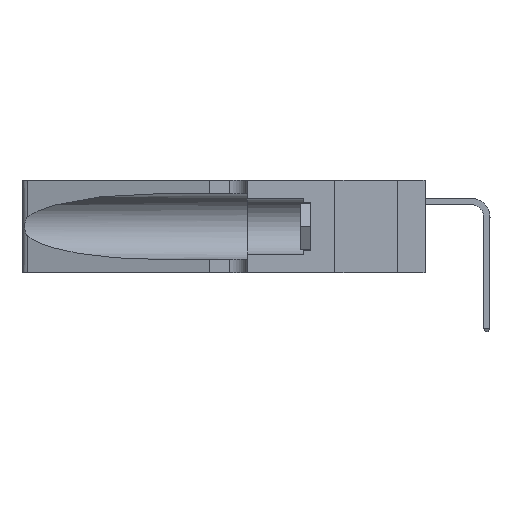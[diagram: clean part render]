
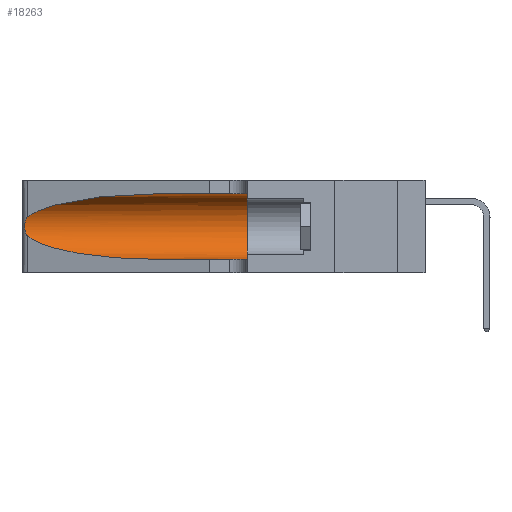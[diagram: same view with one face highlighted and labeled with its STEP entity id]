
A CAD part, left-side view. The second image highlights one B-rep face of the part: STEP entity #18263.
In plain terms, the highlighted cylindrical face has radius 3.308 mm (diameter 6.617 mm), a partial arc.
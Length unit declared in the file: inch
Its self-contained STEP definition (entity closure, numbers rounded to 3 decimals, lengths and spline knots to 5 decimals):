
#2516 = CARTESIAN_POINT ( 'NONE',  ( 0.26075, 1.23896, 0.19203 ) ) ;
#4364 = VERTEX_POINT ( 'NONE', #32372 ) ;
#5464 = CARTESIAN_POINT ( 'NONE',  ( 0.25487, 1.22718, 0.14631 ) ) ;
#6122 = CARTESIAN_POINT ( 'NONE',  ( 0.26017, 1.23833, 0.17102 ) ) ;
#6184 = VERTEX_POINT ( 'NONE', #35176 ) ;
#6889 = CARTESIAN_POINT ( 'NONE',  ( 0.25487, 1.22718, 0.22369 ) ) ;
#7585 = EDGE_CURVE ( 'NONE', #8695, #30227, #9266, .T. ) ;
#8695 = VERTEX_POINT ( 'NONE', #9347 ) ;
#8862 = CARTESIAN_POINT ( 'NONE',  ( 0.1305, 1.61858, 0.05475 ) ) ;
#9090 = CARTESIAN_POINT ( 'NONE',  ( 0.2373, 1.15595, 0.08982 ) ) ;
#9266 = B_SPLINE_CURVE_WITH_KNOTS ( 'NONE', 3,
 ( #16802, #38201, #13188, #20362, #45325, #23944, #2516, #27543, #6122, #31169, #9748, #34754, #13347, #38357 ),
 .UNSPECIFIED., .F., .F.,
 ( 4, 2, 2, 2, 2, 2, 4 ),
 ( 0., 0.00027, 0.00053, 0.00107, 0.0016, 0.00187, 0.00214 ),
 .UNSPECIFIED. ) ;
#9347 = CARTESIAN_POINT ( 'NONE',  ( 0.25487, 1.22718, 0.22369 ) ) ;
#9748 = CARTESIAN_POINT ( 'NONE',  ( 0.25789, 1.23486, 0.15765 ) ) ;
#9821 = VERTEX_POINT ( 'NONE', #20671 ) ;
#10733 = CARTESIAN_POINT ( 'NONE',  ( 0.1305, 0.35, 0.185 ) ) ;
#12693 = CARTESIAN_POINT ( 'NONE',  ( 0.18966, 0.96281, 0.05475 ) ) ;
#13188 = CARTESIAN_POINT ( 'NONE',  ( 0.25639, 1.23184, 0.21858 ) ) ;
#13347 = CARTESIAN_POINT ( 'NONE',  ( 0.25555, 1.22993, 0.14849 ) ) ;
#13577 = EDGE_CURVE ( 'NONE', #30227, #9821, #23516, .T. ) ;
#13754 = AXIS2_PLACEMENT_3D ( 'NONE', #10733, #35727, #14325 ) ;
#14325 = DIRECTION ( 'NONE',  ( 0., 0., 1. ) ) ;
#16802 = CARTESIAN_POINT ( 'NONE',  ( 0.25487, 1.22718, 0.22369 ) ) ;
#16837 = LINE ( 'NONE', #17891, #43051 ) ;
#17891 = CARTESIAN_POINT ( 'NONE',  ( 0.1305, 1.61858, 0.31525 ) ) ;
#18263 = ADVANCED_FACE ( 'NONE', ( #26322 ), #24083, .F. ) ;
#20362 = CARTESIAN_POINT ( 'NONE',  ( 0.25787, 1.23484, 0.2124 ) ) ;
#20671 = CARTESIAN_POINT ( 'NONE',  ( 0.1305, 0.72297, 0.05475 ) ) ;
#21172 = VERTEX_POINT ( 'NONE', #37599 ) ;
#21481 = DIRECTION ( 'NONE',  ( 0., -1., 0. ) ) ;
#21956 = EDGE_CURVE ( 'NONE', #9821, #4364, #39500, .T. ) ;
#22913 = EDGE_CURVE ( 'NONE', #21172, #8695, #27738, .T. ) ;
#23516 =( BOUNDED_CURVE ( )  B_SPLINE_CURVE ( 3, ( #5464, #9090, #12693, #37694 ),
 .UNSPECIFIED., .F., .F. ) 
 B_SPLINE_CURVE_WITH_KNOTS ( ( 4, 4 ),
 ( 3.44316, 4.71239 ),
 .UNSPECIFIED. ) 
 CURVE ( )  GEOMETRIC_REPRESENTATION_ITEM ( )  RATIONAL_B_SPLINE_CURVE ( ( 1., 0.87, 0.87, 1. ) ) 
 REPRESENTATION_ITEM ( '' )  );
#23944 = CARTESIAN_POINT ( 'NONE',  ( 0.26018, 1.23835, 0.19895 ) ) ;
#23991 = ORIENTED_EDGE ( 'NONE', *, *, #37843, .F. ) ;
#24083 = CYLINDRICAL_SURFACE ( 'NONE', #29288, 0.13025 ) ;
#24696 = CARTESIAN_POINT ( 'NONE',  ( 0.1305, 0.72297, 0.31525 ) ) ;
#26322 = FACE_OUTER_BOUND ( 'NONE', #32971, .T. ) ;
#26423 = CARTESIAN_POINT ( 'NONE',  ( 0.25487, 1.22718, 0.14631 ) ) ;
#27321 = ORIENTED_EDGE ( 'NONE', *, *, #13577, .T. ) ;
#27543 = CARTESIAN_POINT ( 'NONE',  ( 0.26075, 1.23896, 0.178 ) ) ;
#27738 =( BOUNDED_CURVE ( )  B_SPLINE_CURVE ( 3, ( #24696, #46072, #28328, #6889 ),
 .UNSPECIFIED., .F., .F. ) 
 B_SPLINE_CURVE_WITH_KNOTS ( ( 4, 4 ),
 ( 1.5708, 2.84003 ),
 .UNSPECIFIED. ) 
 CURVE ( )  GEOMETRIC_REPRESENTATION_ITEM ( )  RATIONAL_B_SPLINE_CURVE ( ( 1., 0.87, 0.87, 1. ) ) 
 REPRESENTATION_ITEM ( '' )  );
#28328 = CARTESIAN_POINT ( 'NONE',  ( 0.2373, 1.15595, 0.28018 ) ) ;
#29288 = AXIS2_PLACEMENT_3D ( 'NONE', #29711, #36878, #36724 ) ;
#29711 = CARTESIAN_POINT ( 'NONE',  ( 0.1305, 1.61858, 0.185 ) ) ;
#30007 = VECTOR ( 'NONE', #37466, 39.37008 ) ;
#30227 = VERTEX_POINT ( 'NONE', #26423 ) ;
#30673 = ORIENTED_EDGE ( 'NONE', *, *, #7585, .T. ) ;
#31169 = CARTESIAN_POINT ( 'NONE',  ( 0.25856, 1.23593, 0.16098 ) ) ;
#32372 = CARTESIAN_POINT ( 'NONE',  ( 0.1305, 0.35, 0.05475 ) ) ;
#32971 = EDGE_LOOP ( 'NONE', ( #44544, #30673, #27321, #38557, #23991, #46327 ) ) ;
#34754 = CARTESIAN_POINT ( 'NONE',  ( 0.25639, 1.23186, 0.15144 ) ) ;
#35176 = CARTESIAN_POINT ( 'NONE',  ( 0.1305, 0.35, 0.31525 ) ) ;
#35727 = DIRECTION ( 'NONE',  ( 0., 1., 0. ) ) ;
#36724 = DIRECTION ( 'NONE',  ( 0., 0., -1. ) ) ;
#36878 = DIRECTION ( 'NONE',  ( 0., -1., 0. ) ) ;
#37466 = DIRECTION ( 'NONE',  ( 0., -1., 0. ) ) ;
#37599 = CARTESIAN_POINT ( 'NONE',  ( 0.1305, 0.72297, 0.31525 ) ) ;
#37694 = CARTESIAN_POINT ( 'NONE',  ( 0.1305, 0.72297, 0.05475 ) ) ;
#37843 = EDGE_CURVE ( 'NONE', #6184, #4364, #45283, .T. ) ;
#37876 = EDGE_CURVE ( 'NONE', #21172, #6184, #16837, .T. ) ;
#38201 = CARTESIAN_POINT ( 'NONE',  ( 0.25555, 1.22994, 0.2215 ) ) ;
#38357 = CARTESIAN_POINT ( 'NONE',  ( 0.25487, 1.22718, 0.14631 ) ) ;
#38557 = ORIENTED_EDGE ( 'NONE', *, *, #21956, .T. ) ;
#39500 = LINE ( 'NONE', #8862, #30007 ) ;
#43051 = VECTOR ( 'NONE', #21481, 39.37008 ) ;
#44544 = ORIENTED_EDGE ( 'NONE', *, *, #22913, .T. ) ;
#45283 = CIRCLE ( 'NONE', #13754, 0.13025 ) ;
#45325 = CARTESIAN_POINT ( 'NONE',  ( 0.25854, 1.2359, 0.20912 ) ) ;
#46072 = CARTESIAN_POINT ( 'NONE',  ( 0.18966, 0.96281, 0.31525 ) ) ;
#46327 = ORIENTED_EDGE ( 'NONE', *, *, #37876, .F. ) ;
